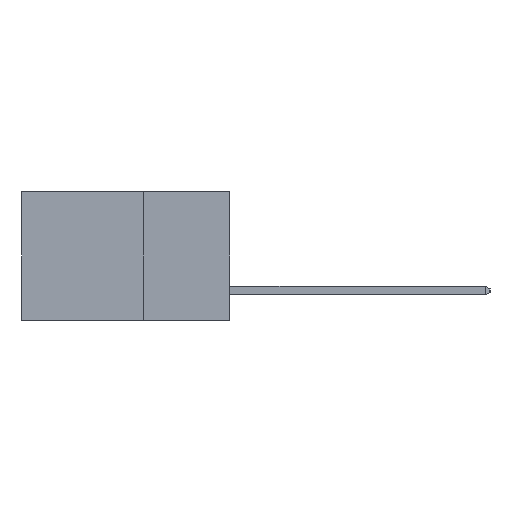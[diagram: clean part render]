
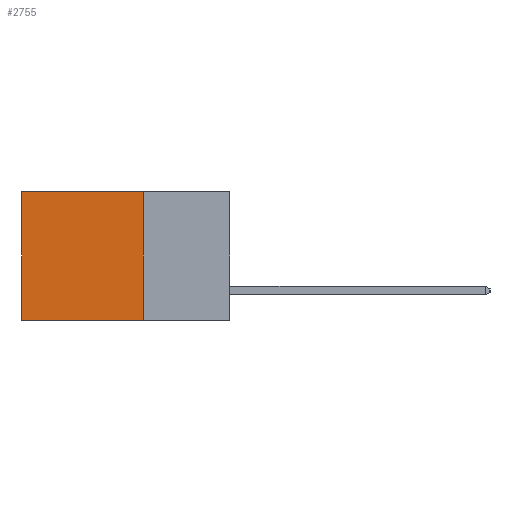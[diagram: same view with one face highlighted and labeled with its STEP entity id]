
A CAD part, left-side view. The second image highlights one B-rep face of the part: STEP entity #2755.
In plain terms, the highlighted planar face has unit normal (-1, 0, 0).
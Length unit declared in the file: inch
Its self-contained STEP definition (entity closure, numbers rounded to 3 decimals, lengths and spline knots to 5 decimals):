
#751 = VERTEX_POINT ( 'NONE', #2001 ) ;
#1348 = CARTESIAN_POINT ( 'NONE',  ( 0.298, 0.25, 0. ) ) ;
#2001 = CARTESIAN_POINT ( 'NONE',  ( 0.298, 0.6, -0.37 ) ) ;
#2047 = VECTOR ( 'NONE', #8540, 39.37008 ) ;
#2128 = ORIENTED_EDGE ( 'NONE', *, *, #2651, .T. ) ;
#2651 = EDGE_CURVE ( 'NONE', #10046, #751, #14903, .T. ) ;
#2755 = ADVANCED_FACE ( 'NONE', ( #5851 ), #3429, .F. ) ;
#3153 = CARTESIAN_POINT ( 'NONE',  ( 0.298, 0.25, 0. ) ) ;
#3429 = PLANE ( 'NONE',  #12238 ) ;
#3567 = VERTEX_POINT ( 'NONE', #1348 ) ;
#4828 = EDGE_CURVE ( 'NONE', #4983, #751, #15647, .T. ) ;
#4983 = VERTEX_POINT ( 'NONE', #10343 ) ;
#5213 = EDGE_CURVE ( 'NONE', #3567, #10046, #10154, .T. ) ;
#5851 = FACE_OUTER_BOUND ( 'NONE', #7472, .T. ) ;
#5996 = DIRECTION ( 'NONE',  ( 0., 0., -1. ) ) ;
#6302 = ORIENTED_EDGE ( 'NONE', *, *, #5213, .T. ) ;
#6622 = ORIENTED_EDGE ( 'NONE', *, *, #17862, .F. ) ;
#7022 = VECTOR ( 'NONE', #5996, 39.37008 ) ;
#7472 = EDGE_LOOP ( 'NONE', ( #2128, #11823, #6622, #6302 ) ) ;
#7648 = VECTOR ( 'NONE', #7762, 39.37008 ) ;
#7762 = DIRECTION ( 'NONE',  ( 0., 0., -1. ) ) ;
#8095 = DIRECTION ( 'NONE',  ( 0., 0., -1. ) ) ;
#8119 = DIRECTION ( 'NONE',  ( 1., 0., 0. ) ) ;
#8323 = CARTESIAN_POINT ( 'NONE',  ( 0.298, 0.25, 0. ) ) ;
#8540 = DIRECTION ( 'NONE',  ( 0., 1., 0. ) ) ;
#8863 = VECTOR ( 'NONE', #11658, 39.37008 ) ;
#10046 = VERTEX_POINT ( 'NONE', #14325 ) ;
#10154 = LINE ( 'NONE', #8323, #2047 ) ;
#10343 = CARTESIAN_POINT ( 'NONE',  ( 0.298, 0.25, -0.37 ) ) ;
#11658 = DIRECTION ( 'NONE',  ( 0., 1., 0. ) ) ;
#11675 = CARTESIAN_POINT ( 'NONE',  ( 0.298, 0.25, -0.37 ) ) ;
#11823 = ORIENTED_EDGE ( 'NONE', *, *, #4828, .F. ) ;
#12238 = AXIS2_PLACEMENT_3D ( 'NONE', #17210, #8119, #8095 ) ;
#14308 = LINE ( 'NONE', #3153, #7022 ) ;
#14325 = CARTESIAN_POINT ( 'NONE',  ( 0.298, 0.6, 0. ) ) ;
#14903 = LINE ( 'NONE', #15005, #7648 ) ;
#15005 = CARTESIAN_POINT ( 'NONE',  ( 0.298, 0.6, 0. ) ) ;
#15647 = LINE ( 'NONE', #11675, #8863 ) ;
#17210 = CARTESIAN_POINT ( 'NONE',  ( 0.298, 0.25, 0. ) ) ;
#17862 = EDGE_CURVE ( 'NONE', #3567, #4983, #14308, .T. ) ;
